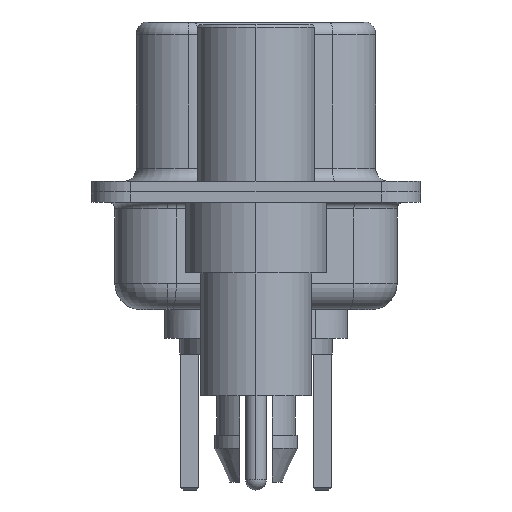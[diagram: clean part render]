
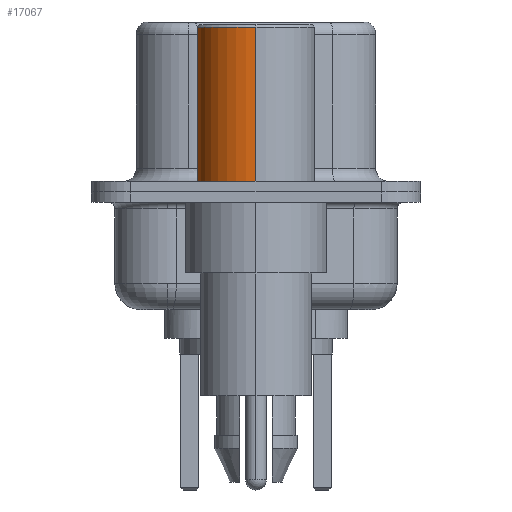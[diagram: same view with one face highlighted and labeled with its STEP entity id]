
A CAD part, left-side view. The second image highlights one B-rep face of the part: STEP entity #17067.
In plain terms, the highlighted cylindrical face has radius 2.25 mm (diameter 4.5 mm), a partial arc.
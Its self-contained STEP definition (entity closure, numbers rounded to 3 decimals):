
#177 = VERTEX_POINT ( 'NONE', #8580 ) ;
#553 = EDGE_CURVE ( 'NONE', #177, #13530, #9584, .T. ) ;
#864 = AXIS2_PLACEMENT_3D ( 'NONE', #11485, #3552, #12805 ) ;
#1090 = VERTEX_POINT ( 'NONE', #1394 ) ;
#1394 = CARTESIAN_POINT ( 'NONE',  ( 2.25, 0., 6.3 ) ) ;
#1729 = EDGE_CURVE ( 'NONE', #13530, #3965, #10563, .T. ) ;
#2312 = DIRECTION ( 'NONE',  ( 0., 0., 1. ) ) ;
#2576 = AXIS2_PLACEMENT_3D ( 'NONE', #14280, #2312, #6417 ) ;
#3185 = EDGE_LOOP ( 'NONE', ( #10203, #4977, #13451, #15848 ) ) ;
#3408 = CARTESIAN_POINT ( 'NONE',  ( -2.25, 0., 6.3 ) ) ;
#3552 = DIRECTION ( 'NONE',  ( 0., 0., 1. ) ) ;
#3965 = VERTEX_POINT ( 'NONE', #3408 ) ;
#4977 = ORIENTED_EDGE ( 'NONE', *, *, #1729, .T. ) ;
#5798 = LINE ( 'NONE', #15527, #12745 ) ;
#6310 = CARTESIAN_POINT ( 'NONE',  ( -2.25, 0., 0.4 ) ) ;
#6417 = DIRECTION ( 'NONE',  ( 1., 0., 0. ) ) ;
#6911 = CARTESIAN_POINT ( 'NONE',  ( 0., 0., 0.4 ) ) ;
#7483 = VECTOR ( 'NONE', #10181, 1000. ) ;
#7965 = CYLINDRICAL_SURFACE ( 'NONE', #2576, 2.25 ) ;
#8580 = CARTESIAN_POINT ( 'NONE',  ( 2.25, 0., 0.4 ) ) ;
#8768 = CARTESIAN_POINT ( 'NONE',  ( -2.25, 0., 0.581 ) ) ;
#8969 = DIRECTION ( 'NONE',  ( 0., 0., 1. ) ) ;
#9584 = CIRCLE ( 'NONE', #10858, 2.25 ) ;
#10181 = DIRECTION ( 'NONE',  ( 0., 0., 1. ) ) ;
#10203 = ORIENTED_EDGE ( 'NONE', *, *, #553, .T. ) ;
#10244 = DIRECTION ( 'NONE',  ( 1., 0., 0. ) ) ;
#10563 = LINE ( 'NONE', #8768, #7483 ) ;
#10847 = CIRCLE ( 'NONE', #864, 2.25 ) ;
#10858 = AXIS2_PLACEMENT_3D ( 'NONE', #6911, #13505, #10244 ) ;
#11485 = CARTESIAN_POINT ( 'NONE',  ( 0., 0., 6.3 ) ) ;
#12745 = VECTOR ( 'NONE', #8969, 1000. ) ;
#12805 = DIRECTION ( 'NONE',  ( 1., 0., 0. ) ) ;
#13451 = ORIENTED_EDGE ( 'NONE', *, *, #16297, .F. ) ;
#13505 = DIRECTION ( 'NONE',  ( 0., 0., 1. ) ) ;
#13530 = VERTEX_POINT ( 'NONE', #6310 ) ;
#14105 = EDGE_CURVE ( 'NONE', #177, #1090, #5798, .T. ) ;
#14280 = CARTESIAN_POINT ( 'NONE',  ( 0., 0., 0.581 ) ) ;
#14963 = FACE_OUTER_BOUND ( 'NONE', #3185, .T. ) ;
#15527 = CARTESIAN_POINT ( 'NONE',  ( 2.25, 0., 0.581 ) ) ;
#15848 = ORIENTED_EDGE ( 'NONE', *, *, #14105, .F. ) ;
#16297 = EDGE_CURVE ( 'NONE', #1090, #3965, #10847, .T. ) ;
#17067 = ADVANCED_FACE ( 'NONE', ( #14963 ), #7965, .T. ) ;
